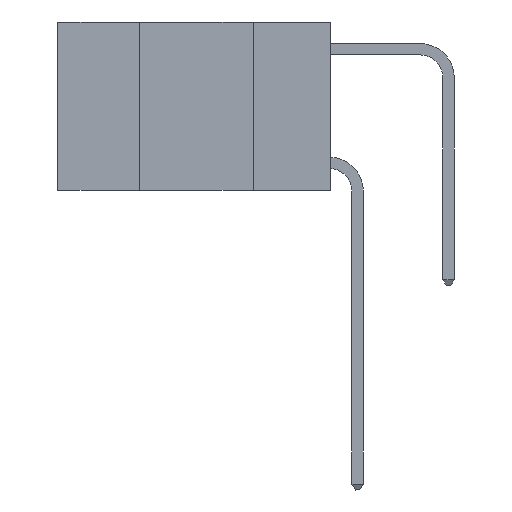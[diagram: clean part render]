
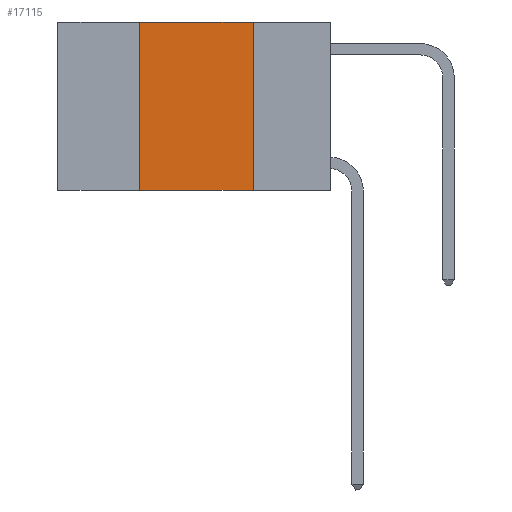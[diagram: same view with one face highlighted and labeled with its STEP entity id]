
A CAD part, left-side view. The second image highlights one B-rep face of the part: STEP entity #17115.
In plain terms, the highlighted planar face has unit normal (-1, 0, 0).
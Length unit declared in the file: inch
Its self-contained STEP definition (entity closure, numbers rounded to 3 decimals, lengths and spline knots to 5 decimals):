
#292 = DIRECTION ( 'NONE',  ( 0., 0., -1. ) ) ;
#867 = CARTESIAN_POINT ( 'NONE',  ( 0., 0.42, 0. ) ) ;
#980 = LINE ( 'NONE', #2379, #3284 ) ;
#2337 = VERTEX_POINT ( 'NONE', #9999 ) ;
#2379 = CARTESIAN_POINT ( 'NONE',  ( 0., 0.42, 0. ) ) ;
#2817 = VERTEX_POINT ( 'NONE', #18265 ) ;
#2900 = EDGE_CURVE ( 'NONE', #2817, #14100, #15524, .T. ) ;
#3284 = VECTOR ( 'NONE', #3996, 39.37008 ) ;
#3996 = DIRECTION ( 'NONE',  ( 0., 0., 1. ) ) ;
#4072 = ORIENTED_EDGE ( 'NONE', *, *, #4415, .F. ) ;
#4289 = VERTEX_POINT ( 'NONE', #867 ) ;
#4415 = EDGE_CURVE ( 'NONE', #2337, #14100, #8957, .T. ) ;
#5285 = VECTOR ( 'NONE', #11201, 39.37008 ) ;
#5456 = CARTESIAN_POINT ( 'NONE',  ( 0., 0.6, 0. ) ) ;
#6581 = VECTOR ( 'NONE', #15348, 39.37008 ) ;
#6682 = LINE ( 'NONE', #5456, #5285 ) ;
#7386 = DIRECTION ( 'NONE',  ( 1., 0., 0. ) ) ;
#7845 = EDGE_CURVE ( 'NONE', #4289, #2337, #6682, .T. ) ;
#8957 = LINE ( 'NONE', #18631, #16524 ) ;
#9435 = ORIENTED_EDGE ( 'NONE', *, *, #2900, .T. ) ;
#9999 = CARTESIAN_POINT ( 'NONE',  ( 0., 0.17, 0. ) ) ;
#10644 = AXIS2_PLACEMENT_3D ( 'NONE', #13019, #7386, #292 ) ;
#11118 = CARTESIAN_POINT ( 'NONE',  ( 0., 0.6, -0.37 ) ) ;
#11201 = DIRECTION ( 'NONE',  ( 0., -1., 0. ) ) ;
#11417 = DIRECTION ( 'NONE',  ( 0., 0., -1. ) ) ;
#11537 = EDGE_CURVE ( 'NONE', #2817, #4289, #980, .T. ) ;
#13019 = CARTESIAN_POINT ( 'NONE',  ( 0., 0.6, 0. ) ) ;
#13027 = EDGE_LOOP ( 'NONE', ( #4072, #18243, #18417, #9435 ) ) ;
#13202 = PLANE ( 'NONE',  #10644 ) ;
#14100 = VERTEX_POINT ( 'NONE', #15289 ) ;
#14539 = FACE_OUTER_BOUND ( 'NONE', #13027, .T. ) ;
#15289 = CARTESIAN_POINT ( 'NONE',  ( 0., 0.17, -0.37 ) ) ;
#15348 = DIRECTION ( 'NONE',  ( 0., -1., 0. ) ) ;
#15524 = LINE ( 'NONE', #11118, #6581 ) ;
#16524 = VECTOR ( 'NONE', #11417, 39.37008 ) ;
#17115 = ADVANCED_FACE ( 'NONE', ( #14539 ), #13202, .F. ) ;
#18243 = ORIENTED_EDGE ( 'NONE', *, *, #7845, .F. ) ;
#18265 = CARTESIAN_POINT ( 'NONE',  ( 0., 0.42, -0.37 ) ) ;
#18417 = ORIENTED_EDGE ( 'NONE', *, *, #11537, .F. ) ;
#18631 = CARTESIAN_POINT ( 'NONE',  ( 0., 0.17, 0. ) ) ;
